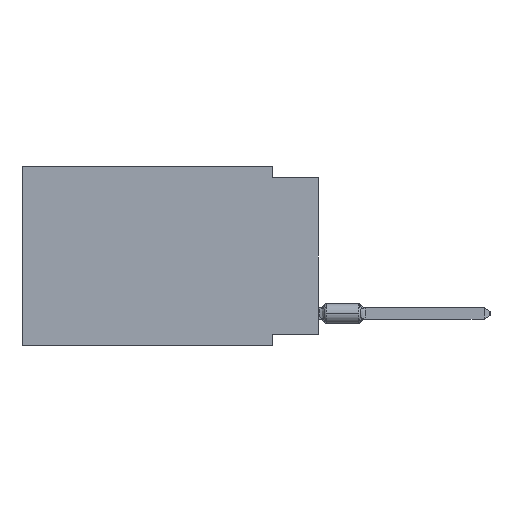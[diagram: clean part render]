
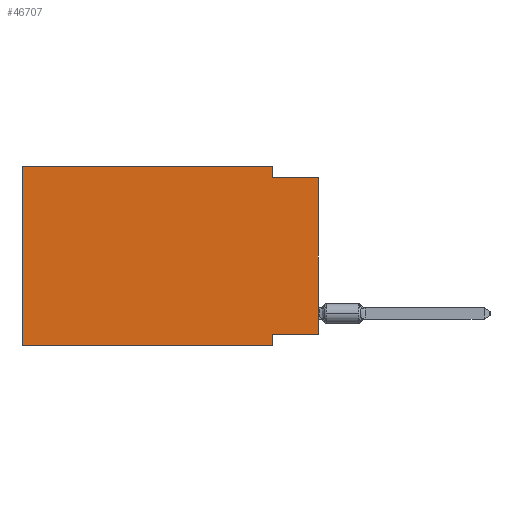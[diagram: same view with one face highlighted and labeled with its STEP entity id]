
A CAD part, left-side view. The second image highlights one B-rep face of the part: STEP entity #46707.
In plain terms, the highlighted planar face has unit normal (-1, 0, 0).
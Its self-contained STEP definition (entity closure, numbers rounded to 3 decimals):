
#1735 = EDGE_CURVE ( 'NONE', #29254, #23957, #10351, .T. ) ;
#1827 = LINE ( 'NONE', #18192, #46292 ) ;
#1904 = EDGE_CURVE ( 'NONE', #58749, #43048, #57939, .T. ) ;
#3262 = VERTEX_POINT ( 'NONE', #36969 ) ;
#3532 = CARTESIAN_POINT ( 'NONE',  ( 0., 16.383, 0. ) ) ;
#4265 = VECTOR ( 'NONE', #31690, 1000. ) ;
#5173 = CARTESIAN_POINT ( 'NONE',  ( 0., 0., -0.635 ) ) ;
#6105 = DIRECTION ( 'NONE',  ( 0., 0., -1. ) ) ;
#10351 = LINE ( 'NONE', #37037, #4265 ) ;
#11893 = CARTESIAN_POINT ( 'NONE',  ( 0., 16.383, -9.906 ) ) ;
#13442 = EDGE_CURVE ( 'NONE', #29254, #3262, #29771, .T. ) ;
#13583 = FACE_OUTER_BOUND ( 'NONE', #44222, .T. ) ;
#14968 = LINE ( 'NONE', #15311, #41953 ) ;
#15311 = CARTESIAN_POINT ( 'NONE',  ( 0., 0., -0.635 ) ) ;
#18192 = CARTESIAN_POINT ( 'NONE',  ( 0., 16.383, -9.906 ) ) ;
#18562 = CARTESIAN_POINT ( 'NONE',  ( 0., 16.383, 0. ) ) ;
#19552 = DIRECTION ( 'NONE',  ( 0., -1., 0. ) ) ;
#19885 = VECTOR ( 'NONE', #51457, 1000. ) ;
#21984 = ORIENTED_EDGE ( 'NONE', *, *, #31801, .F. ) ;
#22372 = CARTESIAN_POINT ( 'NONE',  ( 0., 0., -9.271 ) ) ;
#23528 = CARTESIAN_POINT ( 'NONE',  ( 0., 2.54, -9.906 ) ) ;
#23546 = DIRECTION ( 'NONE',  ( 1., 0., 0. ) ) ;
#23957 = VERTEX_POINT ( 'NONE', #5173 ) ;
#24316 = ORIENTED_EDGE ( 'NONE', *, *, #57599, .F. ) ;
#24799 = LINE ( 'NONE', #46500, #65024 ) ;
#24927 = EDGE_CURVE ( 'NONE', #48321, #58749, #39301, .T. ) ;
#29254 = VERTEX_POINT ( 'NONE', #22372 ) ;
#29771 = LINE ( 'NONE', #31150, #19885 ) ;
#30488 = DIRECTION ( 'NONE',  ( 0., 0., -1. ) ) ;
#31150 = CARTESIAN_POINT ( 'NONE',  ( 0., 0., -9.271 ) ) ;
#31690 = DIRECTION ( 'NONE',  ( 0., 0., 1. ) ) ;
#31801 = EDGE_CURVE ( 'NONE', #36899, #23957, #14968, .T. ) ;
#34453 = EDGE_CURVE ( 'NONE', #43048, #36899, #24799, .T. ) ;
#34567 = VECTOR ( 'NONE', #39652, 1000. ) ;
#35149 = ORIENTED_EDGE ( 'NONE', *, *, #13442, .F. ) ;
#36899 = VERTEX_POINT ( 'NONE', #43080 ) ;
#36929 = DIRECTION ( 'NONE',  ( 0., 0., -1. ) ) ;
#36969 = CARTESIAN_POINT ( 'NONE',  ( 0., 2.54, -9.271 ) ) ;
#37037 = CARTESIAN_POINT ( 'NONE',  ( 0., 0., 0. ) ) ;
#39301 = LINE ( 'NONE', #44631, #34567 ) ;
#39542 = DIRECTION ( 'NONE',  ( 0., -1., 0. ) ) ;
#39652 = DIRECTION ( 'NONE',  ( 0., 0., 1. ) ) ;
#41953 = VECTOR ( 'NONE', #53016, 1000. ) ;
#42819 = VECTOR ( 'NONE', #6105, 1000. ) ;
#43048 = VERTEX_POINT ( 'NONE', #47150 ) ;
#43080 = CARTESIAN_POINT ( 'NONE',  ( 0., 2.54, -0.635 ) ) ;
#44222 = EDGE_LOOP ( 'NONE', ( #61773, #21984, #70012, #69732, #50420, #61405, #24316, #35149 ) ) ;
#44631 = CARTESIAN_POINT ( 'NONE',  ( 0., 16.383, 0. ) ) ;
#44633 = VERTEX_POINT ( 'NONE', #69411 ) ;
#46292 = VECTOR ( 'NONE', #39542, 1000. ) ;
#46500 = CARTESIAN_POINT ( 'NONE',  ( 0., 2.54, 0. ) ) ;
#46707 = ADVANCED_FACE ( 'NONE', ( #13583 ), #58603, .F. ) ;
#47150 = CARTESIAN_POINT ( 'NONE',  ( 0., 2.54, 0. ) ) ;
#48321 = VERTEX_POINT ( 'NONE', #11893 ) ;
#50420 = ORIENTED_EDGE ( 'NONE', *, *, #24927, .F. ) ;
#51111 = CARTESIAN_POINT ( 'NONE',  ( 0., 16.383, 0. ) ) ;
#51457 = DIRECTION ( 'NONE',  ( 0., 1., 0. ) ) ;
#53016 = DIRECTION ( 'NONE',  ( 0., -1., 0. ) ) ;
#55166 = LINE ( 'NONE', #23528, #42819 ) ;
#56530 = VECTOR ( 'NONE', #19552, 1000. ) ;
#56691 = AXIS2_PLACEMENT_3D ( 'NONE', #18562, #23546, #36929 ) ;
#57552 = EDGE_CURVE ( 'NONE', #48321, #44633, #1827, .T. ) ;
#57599 = EDGE_CURVE ( 'NONE', #3262, #44633, #55166, .T. ) ;
#57939 = LINE ( 'NONE', #3532, #56530 ) ;
#58603 = PLANE ( 'NONE',  #56691 ) ;
#58749 = VERTEX_POINT ( 'NONE', #51111 ) ;
#61405 = ORIENTED_EDGE ( 'NONE', *, *, #57552, .T. ) ;
#61773 = ORIENTED_EDGE ( 'NONE', *, *, #1735, .T. ) ;
#65024 = VECTOR ( 'NONE', #30488, 1000. ) ;
#69411 = CARTESIAN_POINT ( 'NONE',  ( 0., 2.54, -9.906 ) ) ;
#69732 = ORIENTED_EDGE ( 'NONE', *, *, #1904, .F. ) ;
#70012 = ORIENTED_EDGE ( 'NONE', *, *, #34453, .F. ) ;
